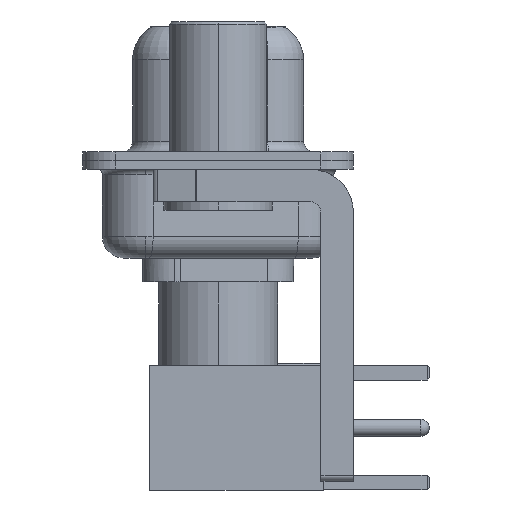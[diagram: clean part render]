
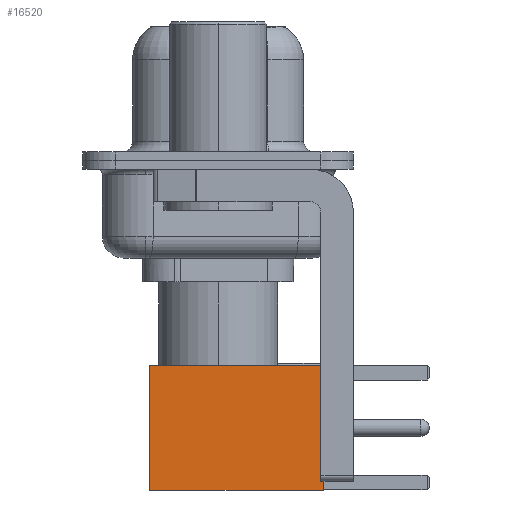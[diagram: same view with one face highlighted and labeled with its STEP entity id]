
A CAD part, left-side view. The second image highlights one B-rep face of the part: STEP entity #16520.
In plain terms, the highlighted face is planar.
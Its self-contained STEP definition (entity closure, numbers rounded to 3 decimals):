
#10 = CARTESIAN_POINT ( 'NONE',  ( 2.875, 2.875, 0. ) ) ;
#379 = DIRECTION ( 'NONE',  ( 0., 0., -1. ) ) ;
#478 = CARTESIAN_POINT ( 'NONE',  ( 0., 2.875, 8. ) ) ;
#593 = LINE ( 'NONE', #478, #19508 ) ;
#2222 = ORIENTED_EDGE ( 'NONE', *, *, #9874, .T. ) ;
#4678 = CARTESIAN_POINT ( 'NONE',  ( 2.875, 2.875, 0. ) ) ;
#5650 = DIRECTION ( 'NONE',  ( -1., 0., 0. ) ) ;
#6481 = EDGE_CURVE ( 'NONE', #11338, #16728, #12760, .T. ) ;
#7032 = CARTESIAN_POINT ( 'NONE',  ( -2.875, 2.875, 0. ) ) ;
#9246 = CARTESIAN_POINT ( 'NONE',  ( 2.875, 2.875, 8. ) ) ;
#9535 = VERTEX_POINT ( 'NONE', #18301 ) ;
#9874 = EDGE_CURVE ( 'NONE', #16728, #9937, #14906, .T. ) ;
#9937 = VERTEX_POINT ( 'NONE', #7032 ) ;
#10101 = PLANE ( 'NONE',  #17324 ) ;
#10216 = DIRECTION ( 'NONE',  ( 0., 0., 1. ) ) ;
#10333 = ORIENTED_EDGE ( 'NONE', *, *, #10373, .F. ) ;
#10373 = EDGE_CURVE ( 'NONE', #9535, #9937, #14021, .T. ) ;
#10937 = CARTESIAN_POINT ( 'NONE',  ( 0., 2.875, 0. ) ) ;
#10978 = VECTOR ( 'NONE', #379, 1000. ) ;
#11338 = VERTEX_POINT ( 'NONE', #9246 ) ;
#11439 = VECTOR ( 'NONE', #17524, 1000. ) ;
#11489 = EDGE_CURVE ( 'NONE', #11338, #9535, #593, .T. ) ;
#11880 = CARTESIAN_POINT ( 'NONE',  ( -2.875, 2.875, 0. ) ) ;
#12760 = LINE ( 'NONE', #16734, #10978 ) ;
#13909 = ORIENTED_EDGE ( 'NONE', *, *, #6481, .T. ) ;
#14021 = LINE ( 'NONE', #11880, #11439 ) ;
#14906 = LINE ( 'NONE', #10937, #19080 ) ;
#15684 = EDGE_LOOP ( 'NONE', ( #13909, #2222, #10333, #17273 ) ) ;
#16520 = ADVANCED_FACE ( 'NONE', ( #23082 ), #10101, .T. ) ;
#16728 = VERTEX_POINT ( 'NONE', #10 ) ;
#16734 = CARTESIAN_POINT ( 'NONE',  ( 2.875, 2.875, 0. ) ) ;
#17273 = ORIENTED_EDGE ( 'NONE', *, *, #11489, .F. ) ;
#17324 = AXIS2_PLACEMENT_3D ( 'NONE', #4678, #21046, #10216 ) ;
#17524 = DIRECTION ( 'NONE',  ( 0., 0., -1. ) ) ;
#18269 = DIRECTION ( 'NONE',  ( -1., 0., 0. ) ) ;
#18301 = CARTESIAN_POINT ( 'NONE',  ( -2.875, 2.875, 8. ) ) ;
#19080 = VECTOR ( 'NONE', #18269, 1000. ) ;
#19508 = VECTOR ( 'NONE', #5650, 1000. ) ;
#21046 = DIRECTION ( 'NONE',  ( 0., 1., 0. ) ) ;
#23082 = FACE_OUTER_BOUND ( 'NONE', #15684, .T. ) ;
